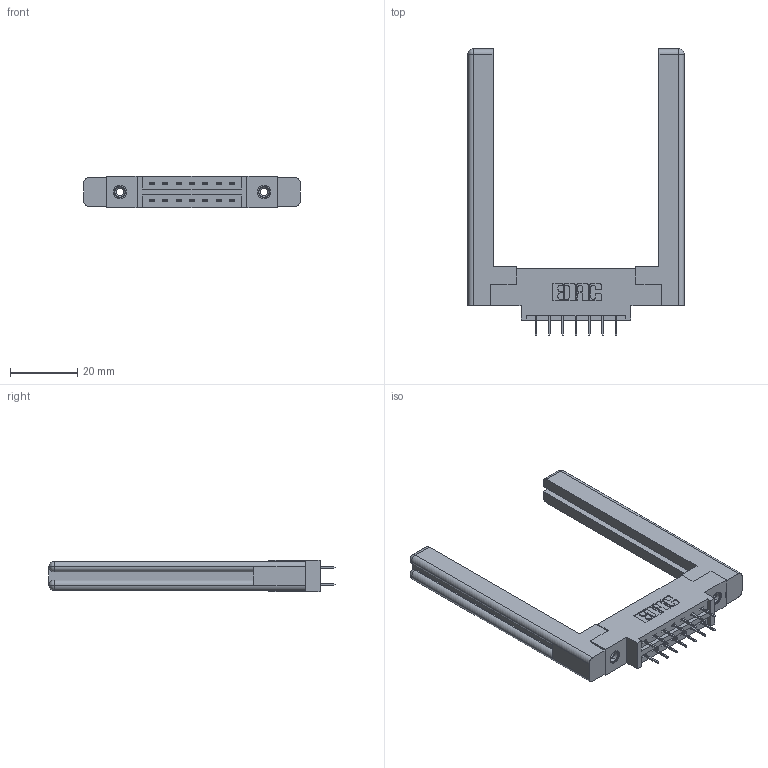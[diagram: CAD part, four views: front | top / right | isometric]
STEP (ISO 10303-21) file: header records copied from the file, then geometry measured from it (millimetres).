
FILE_DESCRIPTION (( 'STEP AP203' ), '1' );
FILE_NAME ('387-014-524-858.STEP', '2019-10-15T21:14:17', ( '' ), ( '' ), 'SwSTEP 2.0', 'SolidWorks 2016', '' );
FILE_SCHEMA (( 'CONFIG_CONTROL_DESIGN' ));
Length unit declared in the file: inch
Products named in the file (5): 307-220-058; 387-014-524-858; 337 Part_0.170 Offset - 0.156 Dia-TI; 345-292-001_345-293-124; 345-250-001_345-250-001-102
Assembly tree (19 placements, depth 2):
  387-014-524-858
    337 Part_0.170 Offset - 0.156 Dia-TI
    345-292-001_345-293-124  x14
    345-250-001_345-250-001-102  x2
    307-220-058  x2
Bounding box: 64.36 x 85.1 x 9.4 mm (x, y, z)
Volume: 13320.9 mm3; surface area: 11733.9 mm2
Topology: 19 solids, 19 shells, 1072 faces, 2987 edges, 1922 vertices
Faces by surface type: plane 774, cylinder 274, cone 12, torus 12
Entity records: 12794 total; most frequent: CARTESIAN_POINT 2193, ORIENTED_EDGE 2068, DIRECTION 1946, EDGE_CURVE 1034, VECTOR 862, LINE 862, VERTEX_POINT 678, AXIS2_PLACEMENT_3D 542
